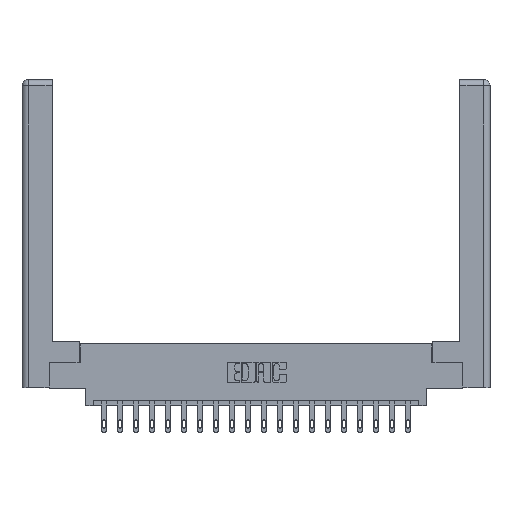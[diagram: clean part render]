
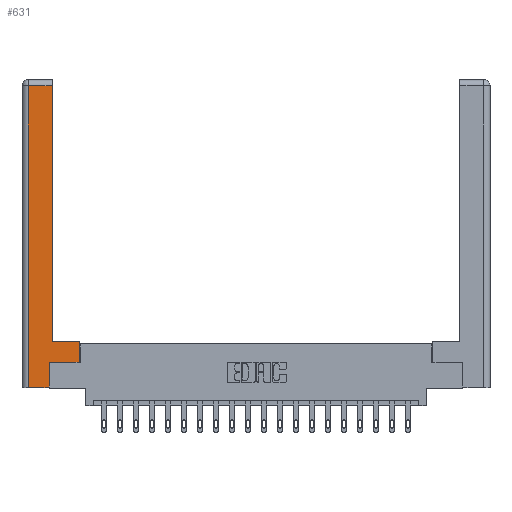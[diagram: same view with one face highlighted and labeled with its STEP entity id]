
A CAD part, top view. The second image highlights one B-rep face of the part: STEP entity #631.
In plain terms, the highlighted planar face has unit normal (0, 0, 1).
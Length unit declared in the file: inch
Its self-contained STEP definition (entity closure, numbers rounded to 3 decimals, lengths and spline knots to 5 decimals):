
#631 = ADVANCED_FACE ( 'NONE', ( #12630 ), #15623, .F. ) ;
#991 = ORIENTED_EDGE ( 'NONE', *, *, #2976, .T. ) ;
#1198 = VECTOR ( 'NONE', #7100, 39.37008 ) ;
#1676 = CARTESIAN_POINT ( 'NONE',  ( 0.0615, 2.94, 0. ) ) ;
#1772 = LINE ( 'NONE', #1676, #9645 ) ;
#2479 = LINE ( 'NONE', #21071, #9332 ) ;
#2558 = VERTEX_POINT ( 'NONE', #8806 ) ;
#2976 = EDGE_CURVE ( 'NONE', #7965, #9260, #2479, .T. ) ;
#3027 = LINE ( 'NONE', #18707, #21051 ) ;
#3629 = EDGE_LOOP ( 'NONE', ( #991, #9746, #8073, #19384, #7123, #10089, #6756, #12275 ) ) ;
#4667 = DIRECTION ( 'NONE',  ( 1., 0., 0. ) ) ;
#4746 = EDGE_CURVE ( 'NONE', #20150, #7965, #9510, .T. ) ;
#5714 = CARTESIAN_POINT ( 'NONE',  ( 0.0615, 2.94, 0. ) ) ;
#6563 = EDGE_CURVE ( 'NONE', #13882, #21048, #10670, .T. ) ;
#6756 = ORIENTED_EDGE ( 'NONE', *, *, #15904, .T. ) ;
#7100 = DIRECTION ( 'NONE',  ( 0., 1., 0. ) ) ;
#7111 = EDGE_CURVE ( 'NONE', #21048, #14231, #14203, .T. ) ;
#7123 = ORIENTED_EDGE ( 'NONE', *, *, #15989, .T. ) ;
#7541 = EDGE_CURVE ( 'NONE', #9260, #13882, #1772, .T. ) ;
#7738 = CARTESIAN_POINT ( 'NONE',  ( 0.295, 0.45, 0. ) ) ;
#7965 = VERTEX_POINT ( 'NONE', #7738 ) ;
#8073 = ORIENTED_EDGE ( 'NONE', *, *, #6563, .T. ) ;
#8720 = DIRECTION ( 'NONE',  ( 0., -1., 0. ) ) ;
#8806 = CARTESIAN_POINT ( 'NONE',  ( 0.265, 0.245, 0. ) ) ;
#8843 = LINE ( 'NONE', #9932, #1198 ) ;
#9260 = VERTEX_POINT ( 'NONE', #11512 ) ;
#9332 = VECTOR ( 'NONE', #11373, 39.37008 ) ;
#9510 = LINE ( 'NONE', #19772, #14310 ) ;
#9543 = AXIS2_PLACEMENT_3D ( 'NONE', #12411, #18320, #19971 ) ;
#9645 = VECTOR ( 'NONE', #14603, 39.37008 ) ;
#9746 = ORIENTED_EDGE ( 'NONE', *, *, #7541, .T. ) ;
#9907 = VECTOR ( 'NONE', #4667, 39.37008 ) ;
#9932 = CARTESIAN_POINT ( 'NONE',  ( 0.265, 0.245, 0. ) ) ;
#10089 = ORIENTED_EDGE ( 'NONE', *, *, #13384, .T. ) ;
#10670 = LINE ( 'NONE', #16046, #20612 ) ;
#11277 = VERTEX_POINT ( 'NONE', #18983 ) ;
#11373 = DIRECTION ( 'NONE',  ( 0., 1., 0. ) ) ;
#11512 = CARTESIAN_POINT ( 'NONE',  ( 0.295, 2.94, 0. ) ) ;
#11867 = VECTOR ( 'NONE', #14684, 39.37008 ) ;
#12275 = ORIENTED_EDGE ( 'NONE', *, *, #4746, .T. ) ;
#12411 = CARTESIAN_POINT ( 'NONE',  ( 0., 0., 0. ) ) ;
#12630 = FACE_OUTER_BOUND ( 'NONE', #3629, .T. ) ;
#13384 = EDGE_CURVE ( 'NONE', #2558, #11277, #3027, .T. ) ;
#13882 = VERTEX_POINT ( 'NONE', #5714 ) ;
#14203 = LINE ( 'NONE', #19215, #9907 ) ;
#14231 = VERTEX_POINT ( 'NONE', #20919 ) ;
#14310 = VECTOR ( 'NONE', #18197, 39.37008 ) ;
#14603 = DIRECTION ( 'NONE',  ( -1., 0., 0. ) ) ;
#14684 = DIRECTION ( 'NONE',  ( 0., 1., 0. ) ) ;
#15623 = PLANE ( 'NONE',  #9543 ) ;
#15769 = CARTESIAN_POINT ( 'NONE',  ( 0.565, 0.45, 0. ) ) ;
#15904 = EDGE_CURVE ( 'NONE', #11277, #20150, #19768, .T. ) ;
#15989 = EDGE_CURVE ( 'NONE', #14231, #2558, #8843, .T. ) ;
#16046 = CARTESIAN_POINT ( 'NONE',  ( 0.0615, 0., 0. ) ) ;
#18014 = CARTESIAN_POINT ( 'NONE',  ( 0.565, 0.45, 0. ) ) ;
#18197 = DIRECTION ( 'NONE',  ( -1., 0., 0. ) ) ;
#18320 = DIRECTION ( 'NONE',  ( 0., 0., -1. ) ) ;
#18707 = CARTESIAN_POINT ( 'NONE',  ( 0.565, 0.245, 0. ) ) ;
#18983 = CARTESIAN_POINT ( 'NONE',  ( 0.565, 0.245, 0. ) ) ;
#19215 = CARTESIAN_POINT ( 'NONE',  ( 0.265, 0., 0. ) ) ;
#19384 = ORIENTED_EDGE ( 'NONE', *, *, #7111, .T. ) ;
#19768 = LINE ( 'NONE', #15769, #11867 ) ;
#19772 = CARTESIAN_POINT ( 'NONE',  ( 0.295, 0.45, 0. ) ) ;
#19971 = DIRECTION ( 'NONE',  ( -1., 0., 0. ) ) ;
#20150 = VERTEX_POINT ( 'NONE', #18014 ) ;
#20231 = DIRECTION ( 'NONE',  ( 1., 0., 0. ) ) ;
#20354 = CARTESIAN_POINT ( 'NONE',  ( 0.0615, 0., 0. ) ) ;
#20612 = VECTOR ( 'NONE', #8720, 39.37008 ) ;
#20919 = CARTESIAN_POINT ( 'NONE',  ( 0.265, 0., 0. ) ) ;
#21048 = VERTEX_POINT ( 'NONE', #20354 ) ;
#21051 = VECTOR ( 'NONE', #20231, 39.37008 ) ;
#21071 = CARTESIAN_POINT ( 'NONE',  ( 0.295, 3., 0. ) ) ;
